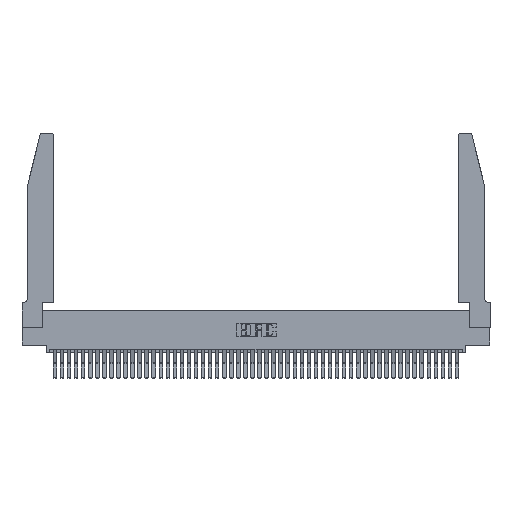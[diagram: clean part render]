
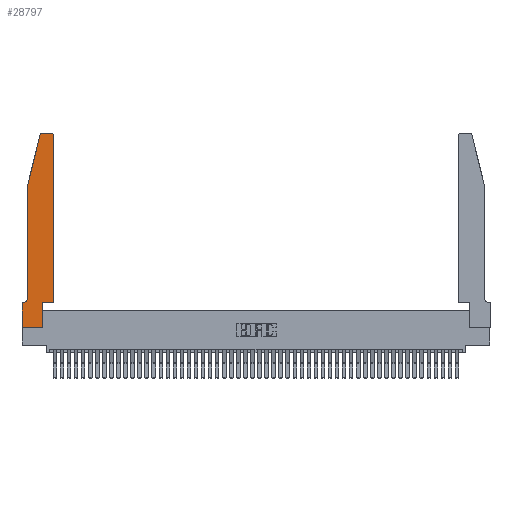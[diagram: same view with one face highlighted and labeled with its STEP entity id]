
A CAD part, top view. The second image highlights one B-rep face of the part: STEP entity #28797.
In plain terms, the highlighted planar face has unit normal (0, 0, 1).
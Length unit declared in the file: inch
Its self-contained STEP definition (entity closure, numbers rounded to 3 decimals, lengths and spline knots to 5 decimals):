
#1372 = VERTEX_POINT ( 'NONE', #6010 ) ;
#1614 = ORIENTED_EDGE ( 'NONE', *, *, #2704, .T. ) ;
#1900 = CARTESIAN_POINT ( 'NONE',  ( 0.0755, 2., 0.37 ) ) ;
#2406 = DIRECTION ( 'NONE',  ( 0., 1., 0. ) ) ;
#2466 = CIRCLE ( 'NONE', #29813, 0.03 ) ;
#2704 = EDGE_CURVE ( 'NONE', #30769, #17050, #47218, .T. ) ;
#2887 = DIRECTION ( 'NONE',  ( 1., 0., 0. ) ) ;
#3787 = AXIS2_PLACEMENT_3D ( 'NONE', #25275, #24947, #2887 ) ;
#5443 = CARTESIAN_POINT ( 'NONE',  ( 0., 0.35, 0.37 ) ) ;
#5448 = DIRECTION ( 'NONE',  ( 0., 0., 1. ) ) ;
#5683 = CARTESIAN_POINT ( 'NONE',  ( 0.0755, 0.42, 0.37 ) ) ;
#6010 = CARTESIAN_POINT ( 'NONE',  ( 0.25487, 2.72718, 0.37 ) ) ;
#6392 = EDGE_LOOP ( 'NONE', ( #30301, #28428, #46781, #9233, #13930, #23893, #7700, #17670, #20053, #44987, #1614, #30160 ) ) ;
#7077 = VERTEX_POINT ( 'NONE', #10699 ) ;
#7098 = CARTESIAN_POINT ( 'NONE',  ( 0.0055, 0.35, 0.37 ) ) ;
#7153 = LINE ( 'NONE', #9588, #45726 ) ;
#7321 = CARTESIAN_POINT ( 'NONE',  ( 0.4505, 0.35, 0.37 ) ) ;
#7700 = ORIENTED_EDGE ( 'NONE', *, *, #28766, .T. ) ;
#7863 = CARTESIAN_POINT ( 'NONE',  ( 0.0755, 2., 0.37 ) ) ;
#7989 = DIRECTION ( 'NONE',  ( 1., 0., 0. ) ) ;
#8630 = CARTESIAN_POINT ( 'NONE',  ( 0.4505, 0.35, 0.37 ) ) ;
#9233 = ORIENTED_EDGE ( 'NONE', *, *, #14662, .T. ) ;
#9588 = CARTESIAN_POINT ( 'NONE',  ( 0.0755, 0.35, 0.37 ) ) ;
#10492 = VERTEX_POINT ( 'NONE', #5683 ) ;
#10699 = CARTESIAN_POINT ( 'NONE',  ( 0.2865, 0.35, 0.37 ) ) ;
#11103 = CIRCLE ( 'NONE', #24543, 0.03 ) ;
#12050 = EDGE_CURVE ( 'NONE', #25304, #47668, #7153, .T. ) ;
#12262 = DIRECTION ( 'NONE',  ( 0., 0., 1. ) ) ;
#12908 = DIRECTION ( 'NONE',  ( -1., 0., 0. ) ) ;
#13930 = ORIENTED_EDGE ( 'NONE', *, *, #19610, .T. ) ;
#14662 = EDGE_CURVE ( 'NONE', #18091, #10492, #25565, .T. ) ;
#16362 = CARTESIAN_POINT ( 'NONE',  ( 0.284, 2.72, 0.37 ) ) ;
#17050 = VERTEX_POINT ( 'NONE', #21884 ) ;
#17633 = DIRECTION ( 'NONE',  ( 0., -1., 0. ) ) ;
#17670 = ORIENTED_EDGE ( 'NONE', *, *, #18454, .T. ) ;
#18091 = VERTEX_POINT ( 'NONE', #7863 ) ;
#18454 = EDGE_CURVE ( 'NONE', #24336, #24800, #26849, .T. ) ;
#18586 = LINE ( 'NONE', #19390, #33798 ) ;
#19390 = CARTESIAN_POINT ( 'NONE',  ( 0., 0., 0.37 ) ) ;
#19610 = EDGE_CURVE ( 'NONE', #10492, #25304, #20868, .T. ) ;
#19651 = LINE ( 'NONE', #47023, #43529 ) ;
#20053 = ORIENTED_EDGE ( 'NONE', *, *, #22748, .T. ) ;
#20378 = LINE ( 'NONE', #1900, #24448 ) ;
#20868 = CIRCLE ( 'NONE', #39105, 0.07 ) ;
#21729 = DIRECTION ( 'NONE',  ( 0., 1., 0. ) ) ;
#21884 = CARTESIAN_POINT ( 'NONE',  ( 0.4505, 2.72, 0.37 ) ) ;
#22748 = EDGE_CURVE ( 'NONE', #24800, #7077, #24082, .T. ) ;
#23888 = VECTOR ( 'NONE', #21729, 39.37008 ) ;
#23893 = ORIENTED_EDGE ( 'NONE', *, *, #12050, .T. ) ;
#24044 = CARTESIAN_POINT ( 'NONE',  ( 0.4205, 2.72, 0.37 ) ) ;
#24082 = LINE ( 'NONE', #28554, #32835 ) ;
#24336 = VERTEX_POINT ( 'NONE', #26707 ) ;
#24448 = VECTOR ( 'NONE', #35902, 39.37008 ) ;
#24543 = AXIS2_PLACEMENT_3D ( 'NONE', #24044, #5448, #42332 ) ;
#24800 = VERTEX_POINT ( 'NONE', #27828 ) ;
#24917 = VERTEX_POINT ( 'NONE', #48180 ) ;
#24947 = DIRECTION ( 'NONE',  ( 0., 0., 1. ) ) ;
#25251 = VECTOR ( 'NONE', #7989, 39.37008 ) ;
#25275 = CARTESIAN_POINT ( 'NONE',  ( 0., 0.35, 0.37 ) ) ;
#25304 = VERTEX_POINT ( 'NONE', #7098 ) ;
#25436 = CARTESIAN_POINT ( 'NONE',  ( 0.284, 2.75, 0.37 ) ) ;
#25565 = LINE ( 'NONE', #39829, #30323 ) ;
#26707 = CARTESIAN_POINT ( 'NONE',  ( 0., 0., 0.37 ) ) ;
#26849 = LINE ( 'NONE', #45242, #40810 ) ;
#27806 = DIRECTION ( 'NONE',  ( -1., 0., 0. ) ) ;
#27828 = CARTESIAN_POINT ( 'NONE',  ( 0.2865, 0., 0.37 ) ) ;
#28412 = EDGE_CURVE ( 'NONE', #1372, #18091, #20378, .T. ) ;
#28428 = ORIENTED_EDGE ( 'NONE', *, *, #37202, .T. ) ;
#28554 = CARTESIAN_POINT ( 'NONE',  ( 0.2865, 0.35, 0.37 ) ) ;
#28766 = EDGE_CURVE ( 'NONE', #47668, #24336, #18586, .T. ) ;
#28797 = ADVANCED_FACE ( 'NONE', ( #34225 ), #47152, .T. ) ;
#29813 = AXIS2_PLACEMENT_3D ( 'NONE', #16362, #12262, #30892 ) ;
#30160 = ORIENTED_EDGE ( 'NONE', *, *, #41044, .T. ) ;
#30301 = ORIENTED_EDGE ( 'NONE', *, *, #35026, .T. ) ;
#30323 = VECTOR ( 'NONE', #17633, 39.37008 ) ;
#30498 = VERTEX_POINT ( 'NONE', #25436 ) ;
#30769 = VERTEX_POINT ( 'NONE', #8630 ) ;
#30892 = DIRECTION ( 'NONE',  ( 1., 0., 0. ) ) ;
#32143 = DIRECTION ( 'NONE',  ( -1., 0., 0. ) ) ;
#32835 = VECTOR ( 'NONE', #2406, 39.37008 ) ;
#33798 = VECTOR ( 'NONE', #34435, 39.37008 ) ;
#34225 = FACE_OUTER_BOUND ( 'NONE', #6392, .T. ) ;
#34435 = DIRECTION ( 'NONE',  ( 0., -1., 0. ) ) ;
#34644 = DIRECTION ( 'NONE',  ( 0., 0., -1. ) ) ;
#35026 = EDGE_CURVE ( 'NONE', #24917, #30498, #19651, .T. ) ;
#35902 = DIRECTION ( 'NONE',  ( -0.239, -0.971, 0. ) ) ;
#37202 = EDGE_CURVE ( 'NONE', #30498, #1372, #2466, .T. ) ;
#37275 = CARTESIAN_POINT ( 'NONE',  ( 0.4505, 0.35, 0.37 ) ) ;
#38552 = CARTESIAN_POINT ( 'NONE',  ( 0.0055, 0.42, 0.37 ) ) ;
#39105 = AXIS2_PLACEMENT_3D ( 'NONE', #38552, #34644, #12908 ) ;
#39819 = LINE ( 'NONE', #7321, #25251 ) ;
#39829 = CARTESIAN_POINT ( 'NONE',  ( 0.0755, 2., 0.37 ) ) ;
#40026 = EDGE_CURVE ( 'NONE', #7077, #30769, #39819, .T. ) ;
#40810 = VECTOR ( 'NONE', #44901, 39.37008 ) ;
#41044 = EDGE_CURVE ( 'NONE', #17050, #24917, #11103, .T. ) ;
#42332 = DIRECTION ( 'NONE',  ( 1., 0., 0. ) ) ;
#43529 = VECTOR ( 'NONE', #27806, 39.37008 ) ;
#44901 = DIRECTION ( 'NONE',  ( 1., 0., 0. ) ) ;
#44987 = ORIENTED_EDGE ( 'NONE', *, *, #40026, .T. ) ;
#45242 = CARTESIAN_POINT ( 'NONE',  ( 0., 0., 0.37 ) ) ;
#45726 = VECTOR ( 'NONE', #32143, 39.37008 ) ;
#46781 = ORIENTED_EDGE ( 'NONE', *, *, #28412, .T. ) ;
#47023 = CARTESIAN_POINT ( 'NONE',  ( 0.2605, 2.75, 0.37 ) ) ;
#47152 = PLANE ( 'NONE',  #3787 ) ;
#47218 = LINE ( 'NONE', #37275, #23888 ) ;
#47668 = VERTEX_POINT ( 'NONE', #5443 ) ;
#48180 = CARTESIAN_POINT ( 'NONE',  ( 0.4205, 2.75, 0.37 ) ) ;
